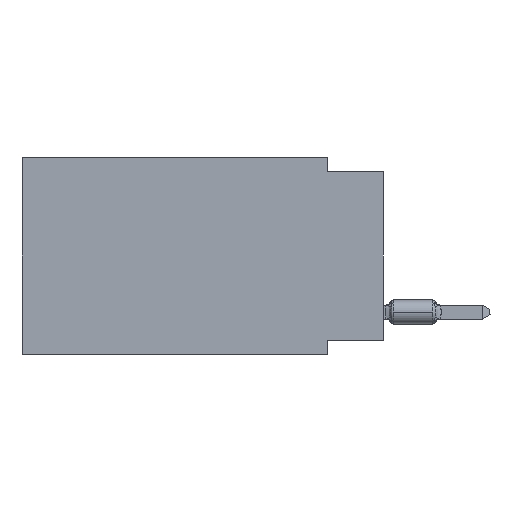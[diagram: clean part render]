
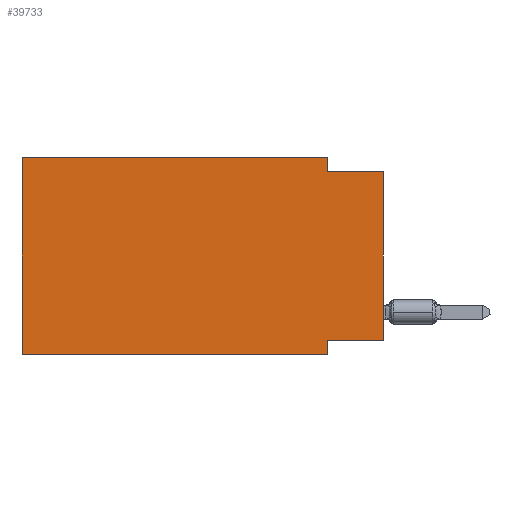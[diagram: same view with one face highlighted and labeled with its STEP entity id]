
A CAD part, left-side view. The second image highlights one B-rep face of the part: STEP entity #39733.
In plain terms, the highlighted planar face has unit normal (-1, 0, 0).
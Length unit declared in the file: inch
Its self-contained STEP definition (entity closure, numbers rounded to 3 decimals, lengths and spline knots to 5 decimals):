
#640 = DIRECTION ( 'NONE',  ( 0., 1., 0. ) ) ;
#846 = DIRECTION ( 'NONE',  ( 0., 0., -1. ) ) ;
#2187 = VERTEX_POINT ( 'NONE', #81867 ) ;
#4596 = DIRECTION ( 'NONE',  ( 0., 0., 1. ) ) ;
#5210 = EDGE_CURVE ( 'NONE', #2187, #61291, #32874, .T. ) ;
#5563 = EDGE_CURVE ( 'NONE', #78031, #40463, #70185, .T. ) ;
#6931 = CARTESIAN_POINT ( 'NONE',  ( 0., 0.1, -0.325 ) ) ;
#8492 = CARTESIAN_POINT ( 'NONE',  ( 0., 0.1, 0. ) ) ;
#8743 = CARTESIAN_POINT ( 'NONE',  ( 0., 0.1, 0. ) ) ;
#9020 = VERTEX_POINT ( 'NONE', #8492 ) ;
#9546 = ORIENTED_EDGE ( 'NONE', *, *, #44294, .F. ) ;
#10200 = PLANE ( 'NONE',  #87578 ) ;
#10791 = VERTEX_POINT ( 'NONE', #65822 ) ;
#12142 = ORIENTED_EDGE ( 'NONE', *, *, #5563, .F. ) ;
#13912 = EDGE_CURVE ( 'NONE', #10791, #40463, #103730, .T. ) ;
#20071 = LINE ( 'NONE', #85396, #59289 ) ;
#21057 = VERTEX_POINT ( 'NONE', #51605 ) ;
#21331 = VECTOR ( 'NONE', #4596, 39.37008 ) ;
#24449 = CARTESIAN_POINT ( 'NONE',  ( 0., 0.645, 0. ) ) ;
#25181 = EDGE_CURVE ( 'NONE', #78421, #61291, #83625, .T. ) ;
#26231 = VECTOR ( 'NONE', #45803, 39.37008 ) ;
#32874 = LINE ( 'NONE', #66014, #68620 ) ;
#34052 = VECTOR ( 'NONE', #846, 39.37008 ) ;
#39733 = ADVANCED_FACE ( 'NONE', ( #66558 ), #10200, .F. ) ;
#40344 = ORIENTED_EDGE ( 'NONE', *, *, #81845, .F. ) ;
#40463 = VERTEX_POINT ( 'NONE', #72219 ) ;
#41839 = DIRECTION ( 'NONE',  ( 0., 0., -1. ) ) ;
#44294 = EDGE_CURVE ( 'NONE', #10791, #21057, #20071, .T. ) ;
#45803 = DIRECTION ( 'NONE',  ( 0., -1., 0. ) ) ;
#46329 = CARTESIAN_POINT ( 'NONE',  ( 0., 0.645, -0.35 ) ) ;
#47369 = CARTESIAN_POINT ( 'NONE',  ( 0., 0., -0.325 ) ) ;
#51605 = CARTESIAN_POINT ( 'NONE',  ( 0., 0.645, 0. ) ) ;
#52204 = DIRECTION ( 'NONE',  ( 0., 0., 1. ) ) ;
#54181 = EDGE_LOOP ( 'NONE', ( #59664, #71998, #98812, #40344, #9546, #102622, #12142, #100394 ) ) ;
#55417 = DIRECTION ( 'NONE',  ( 0., 0., -1. ) ) ;
#57347 = DIRECTION ( 'NONE',  ( 0., -1., 0. ) ) ;
#59167 = DIRECTION ( 'NONE',  ( 0., -1., 0. ) ) ;
#59289 = VECTOR ( 'NONE', #52204, 39.37008 ) ;
#59664 = ORIENTED_EDGE ( 'NONE', *, *, #25181, .T. ) ;
#61291 = VERTEX_POINT ( 'NONE', #64210 ) ;
#62277 = CARTESIAN_POINT ( 'NONE',  ( 0., 0.1, -0.35 ) ) ;
#63265 = EDGE_CURVE ( 'NONE', #9020, #2187, #95696, .T. ) ;
#63879 = CARTESIAN_POINT ( 'NONE',  ( 0., 0., -0.325 ) ) ;
#64210 = CARTESIAN_POINT ( 'NONE',  ( 0., 0., -0.025 ) ) ;
#64560 = EDGE_CURVE ( 'NONE', #78421, #78031, #71777, .T. ) ;
#64730 = CARTESIAN_POINT ( 'NONE',  ( 0., 0.645, 0. ) ) ;
#65748 = LINE ( 'NONE', #64730, #90303 ) ;
#65822 = CARTESIAN_POINT ( 'NONE',  ( 0., 0.645, -0.35 ) ) ;
#66014 = CARTESIAN_POINT ( 'NONE',  ( 0., 0., -0.025 ) ) ;
#66558 = FACE_OUTER_BOUND ( 'NONE', #54181, .T. ) ;
#68620 = VECTOR ( 'NONE', #59167, 39.37008 ) ;
#70185 = LINE ( 'NONE', #62277, #75379 ) ;
#71777 = LINE ( 'NONE', #63879, #86326 ) ;
#71998 = ORIENTED_EDGE ( 'NONE', *, *, #5210, .F. ) ;
#72219 = CARTESIAN_POINT ( 'NONE',  ( 0., 0.1, -0.35 ) ) ;
#72380 = DIRECTION ( 'NONE',  ( 1., 0., 0. ) ) ;
#75379 = VECTOR ( 'NONE', #55417, 39.37008 ) ;
#78031 = VERTEX_POINT ( 'NONE', #6931 ) ;
#78421 = VERTEX_POINT ( 'NONE', #47369 ) ;
#81845 = EDGE_CURVE ( 'NONE', #21057, #9020, #65748, .T. ) ;
#81867 = CARTESIAN_POINT ( 'NONE',  ( 0., 0.1, -0.025 ) ) ;
#83625 = LINE ( 'NONE', #84641, #21331 ) ;
#84641 = CARTESIAN_POINT ( 'NONE',  ( 0., 0., 0. ) ) ;
#85396 = CARTESIAN_POINT ( 'NONE',  ( 0., 0.645, 0. ) ) ;
#86326 = VECTOR ( 'NONE', #640, 39.37008 ) ;
#87578 = AXIS2_PLACEMENT_3D ( 'NONE', #24449, #72380, #41839 ) ;
#90303 = VECTOR ( 'NONE', #57347, 39.37008 ) ;
#95696 = LINE ( 'NONE', #8743, #34052 ) ;
#98812 = ORIENTED_EDGE ( 'NONE', *, *, #63265, .F. ) ;
#100394 = ORIENTED_EDGE ( 'NONE', *, *, #64560, .F. ) ;
#102622 = ORIENTED_EDGE ( 'NONE', *, *, #13912, .T. ) ;
#103730 = LINE ( 'NONE', #46329, #26231 ) ;
